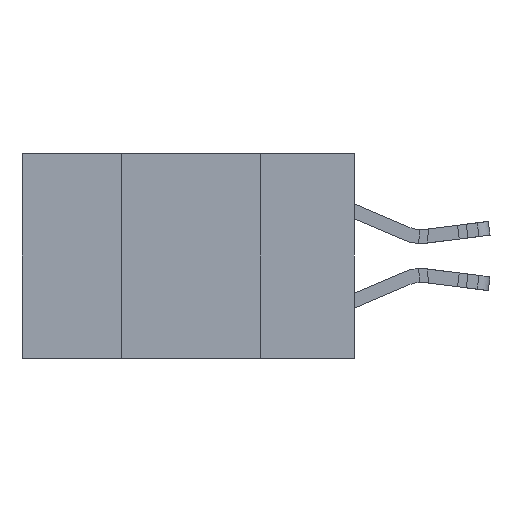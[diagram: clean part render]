
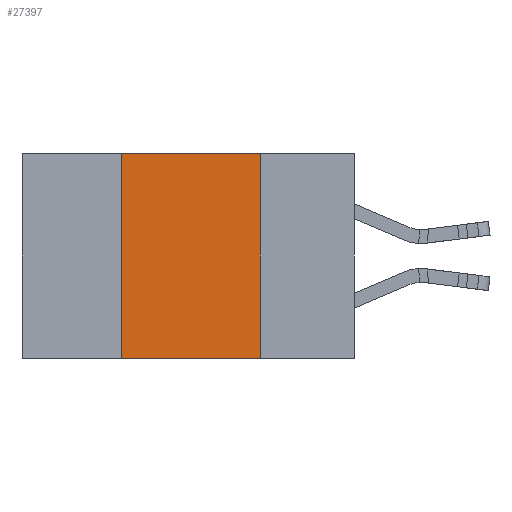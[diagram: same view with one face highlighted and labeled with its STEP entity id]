
A CAD part, left-side view. The second image highlights one B-rep face of the part: STEP entity #27397.
In plain terms, the highlighted planar face has unit normal (-1, 0, 0).
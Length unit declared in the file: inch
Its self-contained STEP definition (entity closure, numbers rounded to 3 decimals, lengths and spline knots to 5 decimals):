
#1055 = CARTESIAN_POINT ( 'NONE',  ( 0., 0.42, 0. ) ) ;
#2668 = DIRECTION ( 'NONE',  ( 0., 0., -1. ) ) ;
#4509 = CARTESIAN_POINT ( 'NONE',  ( 0., 0.17, -0.37 ) ) ;
#5933 = VECTOR ( 'NONE', #19415, 39.37008 ) ;
#6465 = LINE ( 'NONE', #1055, #5933 ) ;
#6669 = VERTEX_POINT ( 'NONE', #15755 ) ;
#6982 = AXIS2_PLACEMENT_3D ( 'NONE', #14076, #16379, #2668 ) ;
#8201 = DIRECTION ( 'NONE',  ( 0., -1., 0. ) ) ;
#9018 = EDGE_LOOP ( 'NONE', ( #14763, #14678, #11296, #9241 ) ) ;
#9241 = ORIENTED_EDGE ( 'NONE', *, *, #12412, .T. ) ;
#9440 = LINE ( 'NONE', #14694, #15917 ) ;
#11296 = ORIENTED_EDGE ( 'NONE', *, *, #16288, .F. ) ;
#12412 = EDGE_CURVE ( 'NONE', #19702, #19336, #18807, .T. ) ;
#12821 = CARTESIAN_POINT ( 'NONE',  ( 0., 0.6, -0.37 ) ) ;
#13079 = CARTESIAN_POINT ( 'NONE',  ( 0., 0.6, 0. ) ) ;
#13175 = DIRECTION ( 'NONE',  ( 0., -1., 0. ) ) ;
#13193 = LINE ( 'NONE', #13079, #27573 ) ;
#14076 = CARTESIAN_POINT ( 'NONE',  ( 0., 0.6, 0. ) ) ;
#14581 = EDGE_CURVE ( 'NONE', #6669, #19336, #9440, .T. ) ;
#14678 = ORIENTED_EDGE ( 'NONE', *, *, #16371, .F. ) ;
#14694 = CARTESIAN_POINT ( 'NONE',  ( 0., 0.17, 0. ) ) ;
#14763 = ORIENTED_EDGE ( 'NONE', *, *, #14581, .F. ) ;
#15755 = CARTESIAN_POINT ( 'NONE',  ( 0., 0.17, 0. ) ) ;
#15917 = VECTOR ( 'NONE', #21549, 39.37008 ) ;
#16288 = EDGE_CURVE ( 'NONE', #19702, #28690, #6465, .T. ) ;
#16371 = EDGE_CURVE ( 'NONE', #28690, #6669, #13193, .T. ) ;
#16379 = DIRECTION ( 'NONE',  ( 1., 0., 0. ) ) ;
#18807 = LINE ( 'NONE', #12821, #19865 ) ;
#18854 = CARTESIAN_POINT ( 'NONE',  ( 0., 0.42, 0. ) ) ;
#19100 = PLANE ( 'NONE',  #6982 ) ;
#19336 = VERTEX_POINT ( 'NONE', #4509 ) ;
#19415 = DIRECTION ( 'NONE',  ( 0., 0., 1. ) ) ;
#19702 = VERTEX_POINT ( 'NONE', #24205 ) ;
#19865 = VECTOR ( 'NONE', #8201, 39.37008 ) ;
#20801 = FACE_OUTER_BOUND ( 'NONE', #9018, .T. ) ;
#21549 = DIRECTION ( 'NONE',  ( 0., 0., -1. ) ) ;
#24205 = CARTESIAN_POINT ( 'NONE',  ( 0., 0.42, -0.37 ) ) ;
#27397 = ADVANCED_FACE ( 'NONE', ( #20801 ), #19100, .F. ) ;
#27573 = VECTOR ( 'NONE', #13175, 39.37008 ) ;
#28690 = VERTEX_POINT ( 'NONE', #18854 ) ;
